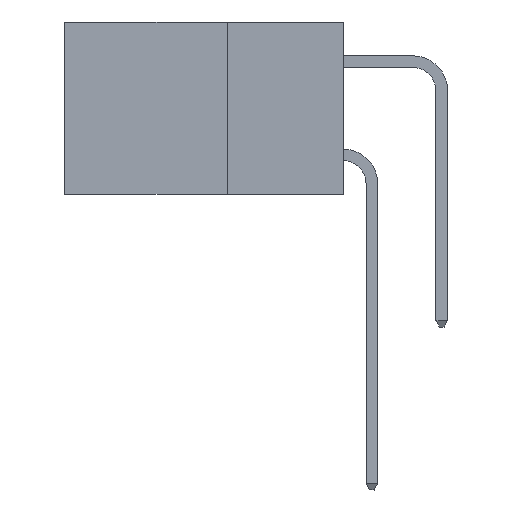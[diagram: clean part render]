
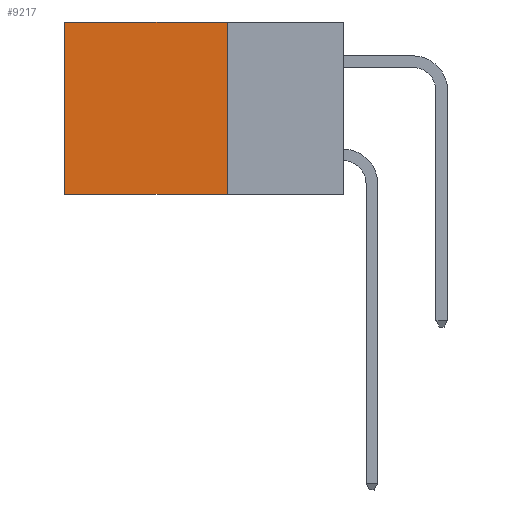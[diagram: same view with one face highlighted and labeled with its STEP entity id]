
A CAD part, left-side view. The second image highlights one B-rep face of the part: STEP entity #9217.
In plain terms, the highlighted planar face has unit normal (-1, 0, 0).
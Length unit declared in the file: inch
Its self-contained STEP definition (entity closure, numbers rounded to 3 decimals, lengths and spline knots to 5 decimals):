
#298 = EDGE_CURVE ( 'NONE', #3247, #2872, #4106, .T. ) ;
#493 = LINE ( 'NONE', #7611, #11250 ) ;
#1218 = CARTESIAN_POINT ( 'NONE',  ( 0.298, 0.25, -0.37 ) ) ;
#1739 = CARTESIAN_POINT ( 'NONE',  ( 0.298, 0.25, 0. ) ) ;
#1937 = CARTESIAN_POINT ( 'NONE',  ( 0.298, 0.6, -0.37 ) ) ;
#2044 = DIRECTION ( 'NONE',  ( 0., 0., -1. ) ) ;
#2055 = CARTESIAN_POINT ( 'NONE',  ( 0.298, 0.6, 0. ) ) ;
#2739 = LINE ( 'NONE', #2055, #7871 ) ;
#2872 = VERTEX_POINT ( 'NONE', #7419 ) ;
#3117 = VERTEX_POINT ( 'NONE', #1937 ) ;
#3247 = VERTEX_POINT ( 'NONE', #1739 ) ;
#3558 = EDGE_CURVE ( 'NONE', #3247, #6768, #493, .T. ) ;
#4106 = LINE ( 'NONE', #11752, #9124 ) ;
#4496 = PLANE ( 'NONE',  #7459 ) ;
#4709 = ORIENTED_EDGE ( 'NONE', *, *, #6520, .T. ) ;
#5242 = FACE_OUTER_BOUND ( 'NONE', #8346, .T. ) ;
#6520 = EDGE_CURVE ( 'NONE', #2872, #3117, #2739, .T. ) ;
#6720 = DIRECTION ( 'NONE',  ( 0., 1., 0. ) ) ;
#6768 = VERTEX_POINT ( 'NONE', #1218 ) ;
#6824 = DIRECTION ( 'NONE',  ( 0., 1., 0. ) ) ;
#6854 = CARTESIAN_POINT ( 'NONE',  ( 0.298, 0.25, 0. ) ) ;
#7023 = VECTOR ( 'NONE', #6824, 39.37008 ) ;
#7419 = CARTESIAN_POINT ( 'NONE',  ( 0.298, 0.6, 0. ) ) ;
#7459 = AXIS2_PLACEMENT_3D ( 'NONE', #6854, #12407, #12077 ) ;
#7611 = CARTESIAN_POINT ( 'NONE',  ( 0.298, 0.25, 0. ) ) ;
#7871 = VECTOR ( 'NONE', #2044, 39.37008 ) ;
#8002 = EDGE_CURVE ( 'NONE', #6768, #3117, #9931, .T. ) ;
#8346 = EDGE_LOOP ( 'NONE', ( #4709, #10210, #10227, #11367 ) ) ;
#9124 = VECTOR ( 'NONE', #6720, 39.37008 ) ;
#9217 = ADVANCED_FACE ( 'NONE', ( #5242 ), #4496, .F. ) ;
#9931 = LINE ( 'NONE', #12833, #7023 ) ;
#10152 = DIRECTION ( 'NONE',  ( 0., 0., -1. ) ) ;
#10210 = ORIENTED_EDGE ( 'NONE', *, *, #8002, .F. ) ;
#10227 = ORIENTED_EDGE ( 'NONE', *, *, #3558, .F. ) ;
#11250 = VECTOR ( 'NONE', #10152, 39.37008 ) ;
#11367 = ORIENTED_EDGE ( 'NONE', *, *, #298, .T. ) ;
#11752 = CARTESIAN_POINT ( 'NONE',  ( 0.298, 0.25, 0. ) ) ;
#12077 = DIRECTION ( 'NONE',  ( 0., 0., -1. ) ) ;
#12407 = DIRECTION ( 'NONE',  ( 1., 0., 0. ) ) ;
#12833 = CARTESIAN_POINT ( 'NONE',  ( 0.298, 0.25, -0.37 ) ) ;
